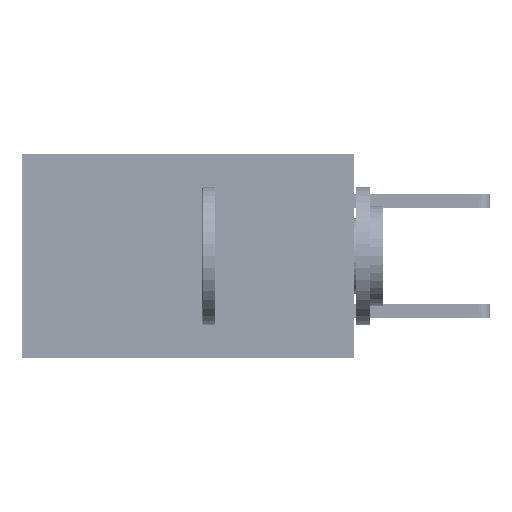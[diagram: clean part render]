
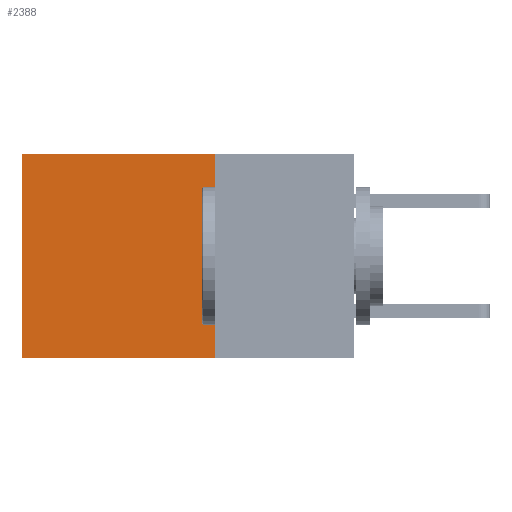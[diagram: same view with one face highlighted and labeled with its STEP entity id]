
A CAD part, left-side view. The second image highlights one B-rep face of the part: STEP entity #2388.
In plain terms, the highlighted planar face has unit normal (-1, 0, 0).
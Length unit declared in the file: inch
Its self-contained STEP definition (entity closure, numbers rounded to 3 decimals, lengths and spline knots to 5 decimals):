
#1668 = CARTESIAN_POINT ( 'NONE',  ( 0.2875, 0.25, 0. ) ) ;
#2143 = CARTESIAN_POINT ( 'NONE',  ( 0.2875, 0.25, 0. ) ) ;
#2388 = ADVANCED_FACE ( 'NONE', ( #22247 ), #17720, .F. ) ;
#5600 = VECTOR ( 'NONE', #36922, 39.37008 ) ;
#5830 = VERTEX_POINT ( 'NONE', #26413 ) ;
#6466 = ORIENTED_EDGE ( 'NONE', *, *, #29109, .T. ) ;
#8157 = VERTEX_POINT ( 'NONE', #27916 ) ;
#9457 = LINE ( 'NONE', #38188, #22237 ) ;
#13709 = CARTESIAN_POINT ( 'NONE',  ( 0.2875, 0.6, 0. ) ) ;
#13982 = DIRECTION ( 'NONE',  ( 0., 0., -1. ) ) ;
#14444 = VECTOR ( 'NONE', #40888, 39.37008 ) ;
#14854 = EDGE_CURVE ( 'NONE', #49454, #8157, #43977, .T. ) ;
#14882 = DIRECTION ( 'NONE',  ( 0., 1., 0. ) ) ;
#14986 = CARTESIAN_POINT ( 'NONE',  ( 0.2875, 0.25, 0. ) ) ;
#15209 = ORIENTED_EDGE ( 'NONE', *, *, #44073, .T. ) ;
#15236 = CARTESIAN_POINT ( 'NONE',  ( 0.2875, 0.25, -0.37 ) ) ;
#15516 = AXIS2_PLACEMENT_3D ( 'NONE', #2143, #37218, #13982 ) ;
#17720 = PLANE ( 'NONE',  #15516 ) ;
#18660 = CARTESIAN_POINT ( 'NONE',  ( 0.2875, 0.6, -0.37 ) ) ;
#20189 = VERTEX_POINT ( 'NONE', #18660 ) ;
#22237 = VECTOR ( 'NONE', #22725, 39.37008 ) ;
#22247 = FACE_OUTER_BOUND ( 'NONE', #36409, .T. ) ;
#22725 = DIRECTION ( 'NONE',  ( 0., 1., 0. ) ) ;
#26413 = CARTESIAN_POINT ( 'NONE',  ( 0.2875, 0.6, 0. ) ) ;
#27916 = CARTESIAN_POINT ( 'NONE',  ( 0.2875, 0.25, -0.37 ) ) ;
#28576 = ORIENTED_EDGE ( 'NONE', *, *, #14854, .F. ) ;
#29109 = EDGE_CURVE ( 'NONE', #49454, #5830, #9457, .T. ) ;
#31932 = EDGE_CURVE ( 'NONE', #8157, #20189, #41950, .T. ) ;
#35100 = LINE ( 'NONE', #13709, #14444 ) ;
#36409 = EDGE_LOOP ( 'NONE', ( #15209, #45305, #28576, #6466 ) ) ;
#36922 = DIRECTION ( 'NONE',  ( 0., 0., -1. ) ) ;
#37218 = DIRECTION ( 'NONE',  ( 1., 0., 0. ) ) ;
#38188 = CARTESIAN_POINT ( 'NONE',  ( 0.2875, 0.25, 0. ) ) ;
#40888 = DIRECTION ( 'NONE',  ( 0., 0., -1. ) ) ;
#41950 = LINE ( 'NONE', #15236, #48643 ) ;
#43977 = LINE ( 'NONE', #1668, #5600 ) ;
#44073 = EDGE_CURVE ( 'NONE', #5830, #20189, #35100, .T. ) ;
#45305 = ORIENTED_EDGE ( 'NONE', *, *, #31932, .F. ) ;
#48643 = VECTOR ( 'NONE', #14882, 39.37008 ) ;
#49454 = VERTEX_POINT ( 'NONE', #14986 ) ;
